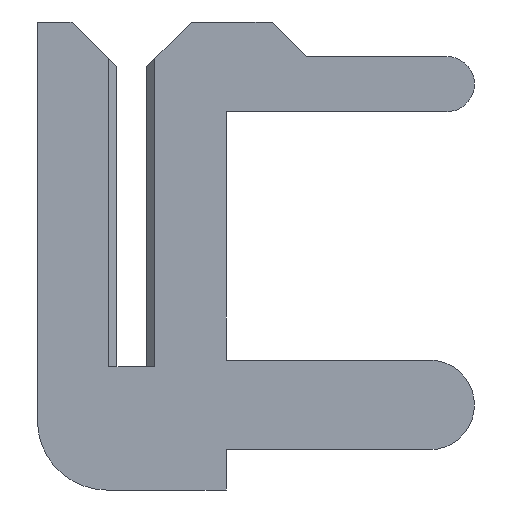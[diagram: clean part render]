
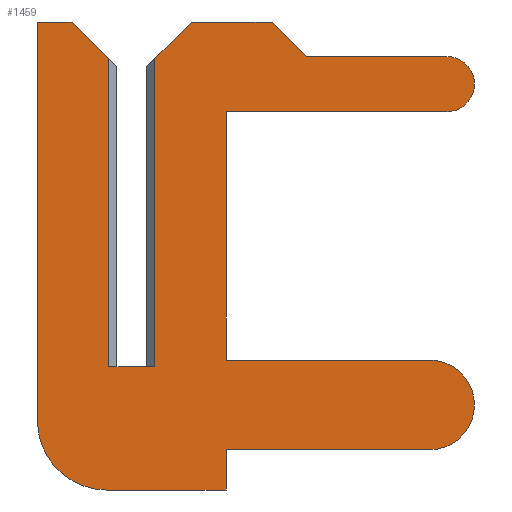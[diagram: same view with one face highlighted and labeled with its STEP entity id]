
A CAD part, left-side view. The second image highlights one B-rep face of the part: STEP entity #1459.
In plain terms, the highlighted planar face has unit normal (-1, 0, 0).
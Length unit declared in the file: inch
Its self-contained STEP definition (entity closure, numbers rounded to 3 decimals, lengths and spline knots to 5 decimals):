
#19 = ORIENTED_EDGE ( 'NONE', *, *, #220, .F. ) ;
#20 = CARTESIAN_POINT ( 'NONE',  ( -0.01, 0.01, 0. ) ) ;
#39 = CARTESIAN_POINT ( 'NONE',  ( -0.01, -0.1295, -0.0165 ) ) ;
#45 = VECTOR ( 'NONE', #202, 39.37008 ) ;
#55 = DIRECTION ( 'NONE',  ( 0., 0., 1. ) ) ;
#58 = ORIENTED_EDGE ( 'NONE', *, *, #839, .F. ) ;
#74 = EDGE_CURVE ( 'NONE', #909, #500, #1623, .T. ) ;
#92 = EDGE_CURVE ( 'NONE', #424, #322, #1539, .T. ) ;
#100 = VERTEX_POINT ( 'NONE', #1485 ) ;
#109 = CARTESIAN_POINT ( 'NONE',  ( -0.01, 0.0065, 0. ) ) ;
#128 = LINE ( 'NONE', #1517, #898 ) ;
#144 = VERTEX_POINT ( 'NONE', #276 ) ;
#150 = CARTESIAN_POINT ( 'NONE',  ( -0.01, 0.011, -0.0235 ) ) ;
#162 = VECTOR ( 'NONE', #884, 39.37008 ) ;
#175 = CARTESIAN_POINT ( 'NONE',  ( -0.01, -0.076, 0.135 ) ) ;
#179 = DIRECTION ( 'NONE',  ( 0., 0., -1. ) ) ;
#187 = EDGE_CURVE ( 'NONE', #1554, #996, #305, .T. ) ;
#195 = VECTOR ( 'NONE', #868, 39.37008 ) ;
#202 = DIRECTION ( 'NONE',  ( 0., -1., 0. ) ) ;
#220 = EDGE_CURVE ( 'NONE', #574, #391, #1400, .T. ) ;
#236 = VECTOR ( 'NONE', #342, 39.37008 ) ;
#249 = CARTESIAN_POINT ( 'NONE',  ( -0.01, 0.01, 0.134 ) ) ;
#250 = EDGE_CURVE ( 'NONE', #1470, #949, #1541, .T. ) ;
#256 = LINE ( 'NONE', #485, #236 ) ;
#273 = DIRECTION ( 'NONE',  ( 0., -0.707, -0.707 ) ) ;
#276 = CARTESIAN_POINT ( 'NONE',  ( -0.01, 0.026, 0.15 ) ) ;
#294 = DIRECTION ( 'NONE',  ( -1., 0., 0. ) ) ;
#298 = CARTESIAN_POINT ( 'NONE',  ( -0.01, -0.137, 0.123 ) ) ;
#305 = LINE ( 'NONE', #721, #1479 ) ;
#308 = DIRECTION ( 'NONE',  ( 0., 1., 0. ) ) ;
#322 = VERTEX_POINT ( 'NONE', #470 ) ;
#342 = DIRECTION ( 'NONE',  ( 0., -1., 0. ) ) ;
#343 = LINE ( 'NONE', #1061, #616 ) ;
#367 = LINE ( 'NONE', #109, #162 ) ;
#370 = EDGE_CURVE ( 'NONE', #996, #1699, #1678, .T. ) ;
#389 = ORIENTED_EDGE ( 'NONE', *, *, #857, .F. ) ;
#391 = VERTEX_POINT ( 'NONE', #599 ) ;
#394 = EDGE_CURVE ( 'NONE', #391, #1491, #128, .T. ) ;
#402 = VERTEX_POINT ( 'NONE', #175 ) ;
#406 = EDGE_CURVE ( 'NONE', #500, #1367, #1132, .T. ) ;
#419 = DIRECTION ( 'NONE',  ( 0., -0.707, -0.707 ) ) ;
#424 = VERTEX_POINT ( 'NONE', #1506 ) ;
#434 = LINE ( 'NONE', #876, #1455 ) ;
#441 = EDGE_CURVE ( 'NONE', #1434, #1015, #557, .T. ) ;
#447 = AXIS2_PLACEMENT_3D ( 'NONE', #1046, #1684, #1445 ) ;
#450 = DIRECTION ( 'NONE',  ( 0., 0., 1. ) ) ;
#451 = ORIENTED_EDGE ( 'NONE', *, *, #92, .T. ) ;
#470 = CARTESIAN_POINT ( 'NONE',  ( -0.01, -0.01, 0. ) ) ;
#485 = CARTESIAN_POINT ( 'NONE',  ( -0.01, -0.137, 0.135 ) ) ;
#500 = VERTEX_POINT ( 'NONE', #1148 ) ;
#511 = ORIENTED_EDGE ( 'NONE', *, *, #820, .F. ) ;
#533 = CARTESIAN_POINT ( 'NONE',  ( -0.01, -0.041, 0.003 ) ) ;
#551 = EDGE_CURVE ( 'NONE', #402, #909, #256, .T. ) ;
#557 = LINE ( 'NONE', #596, #195 ) ;
#558 = DIRECTION ( 'NONE',  ( 1., 0., 0. ) ) ;
#574 = VERTEX_POINT ( 'NONE', #1524 ) ;
#575 = CARTESIAN_POINT ( 'NONE',  ( -0.01, 0.011, -0.0535 ) ) ;
#595 = ORIENTED_EDGE ( 'NONE', *, *, #370, .F. ) ;
#596 = CARTESIAN_POINT ( 'NONE',  ( -0.01, -0.026, 0.15 ) ) ;
#599 = CARTESIAN_POINT ( 'NONE',  ( -0.01, -0.041, -0.0535 ) ) ;
#603 = AXIS2_PLACEMENT_3D ( 'NONE', #298, #558, #1094 ) ;
#610 = ORIENTED_EDGE ( 'NONE', *, *, #1169, .F. ) ;
#614 = VECTOR ( 'NONE', #1592, 39.37008 ) ;
#616 = VECTOR ( 'NONE', #273, 39.37008 ) ;
#641 = EDGE_LOOP ( 'NONE', ( #58, #451, #511, #794, #1536, #1165, #389, #1477, #869, #19, #690, #595, #672, #1370, #1292, #1181, #912, #610, #1146 ) ) ;
#655 = LINE ( 'NONE', #1009, #45 ) ;
#672 = ORIENTED_EDGE ( 'NONE', *, *, #187, .F. ) ;
#675 = CARTESIAN_POINT ( 'NONE',  ( -0.01, -0.041, -0.0535 ) ) ;
#677 = CARTESIAN_POINT ( 'NONE',  ( -0.01, -0.041, 0.003 ) ) ;
#690 = ORIENTED_EDGE ( 'NONE', *, *, #720, .F. ) ;
#698 = DIRECTION ( 'NONE',  ( 0., 1., 0. ) ) ;
#717 = LINE ( 'NONE', #1159, #855 ) ;
#720 = EDGE_CURVE ( 'NONE', #1699, #574, #434, .T. ) ;
#721 = CARTESIAN_POINT ( 'NONE',  ( -0.01, -0.1295, 0.003 ) ) ;
#759 = CARTESIAN_POINT ( 'NONE',  ( -0.01, -0.061, 0.15 ) ) ;
#765 = AXIS2_PLACEMENT_3D ( 'NONE', #39, #971, #450 ) ;
#773 = LINE ( 'NONE', #533, #1433 ) ;
#780 = EDGE_CURVE ( 'NONE', #100, #144, #655, .T. ) ;
#792 = LINE ( 'NONE', #922, #1275 ) ;
#794 = ORIENTED_EDGE ( 'NONE', *, *, #250, .T. ) ;
#801 = DIRECTION ( 'NONE',  ( 0., 0., -1. ) ) ;
#820 = EDGE_CURVE ( 'NONE', #1470, #322, #367, .T. ) ;
#839 = EDGE_CURVE ( 'NONE', #424, #1434, #717, .T. ) ;
#855 = VECTOR ( 'NONE', #1698, 39.37008 ) ;
#857 = EDGE_CURVE ( 'NONE', #1520, #100, #1025, .T. ) ;
#859 = DIRECTION ( 'NONE',  ( 0., 1., 0. ) ) ;
#868 = DIRECTION ( 'NONE',  ( 0., -1., 0. ) ) ;
#869 = ORIENTED_EDGE ( 'NONE', *, *, #394, .F. ) ;
#876 = CARTESIAN_POINT ( 'NONE',  ( -0.01, -0.041, -0.036 ) ) ;
#884 = DIRECTION ( 'NONE',  ( 0., -1., 0. ) ) ;
#898 = VECTOR ( 'NONE', #698, 39.37008 ) ;
#907 = DIRECTION ( 'NONE',  ( 0., 0., 1. ) ) ;
#909 = VERTEX_POINT ( 'NONE', #1551 ) ;
#912 = ORIENTED_EDGE ( 'NONE', *, *, #551, .F. ) ;
#922 = CARTESIAN_POINT ( 'NONE',  ( -0.01, -0.076, 0.135 ) ) ;
#935 = VECTOR ( 'NONE', #907, 39.37008 ) ;
#941 = CARTESIAN_POINT ( 'NONE',  ( -0.01, 0.041, -0.0235 ) ) ;
#947 = PLANE ( 'NONE',  #1156 ) ;
#949 = VERTEX_POINT ( 'NONE', #249 ) ;
#966 = VECTOR ( 'NONE', #308, 39.37008 ) ;
#971 = DIRECTION ( 'NONE',  ( 1., 0., 0. ) ) ;
#981 = CARTESIAN_POINT ( 'NONE',  ( -0.01, -0.041, 0.111 ) ) ;
#996 = VERTEX_POINT ( 'NONE', #1680 ) ;
#1008 = FACE_OUTER_BOUND ( 'NONE', #641, .T. ) ;
#1009 = CARTESIAN_POINT ( 'NONE',  ( -0.01, 0.026, 0.15 ) ) ;
#1015 = VERTEX_POINT ( 'NONE', #759 ) ;
#1025 = LINE ( 'NONE', #1557, #935 ) ;
#1046 = CARTESIAN_POINT ( 'NONE',  ( -0.01, 0.011, -0.0235 ) ) ;
#1047 = VECTOR ( 'NONE', #55, 39.37008 ) ;
#1050 = EDGE_CURVE ( 'NONE', #1491, #1520, #1208, .T. ) ;
#1061 = CARTESIAN_POINT ( 'NONE',  ( -0.01, 0.0065, 0.1305 ) ) ;
#1076 = CARTESIAN_POINT ( 'NONE',  ( -0.01, -0.01, 0.15 ) ) ;
#1090 = CARTESIAN_POINT ( 'NONE',  ( -0.01, -0.041, 0.111 ) ) ;
#1094 = DIRECTION ( 'NONE',  ( 0., 0., 1. ) ) ;
#1132 = LINE ( 'NONE', #981, #966 ) ;
#1142 = EDGE_CURVE ( 'NONE', #1367, #1554, #773, .T. ) ;
#1146 = ORIENTED_EDGE ( 'NONE', *, *, #441, .F. ) ;
#1148 = CARTESIAN_POINT ( 'NONE',  ( -0.01, -0.137, 0.111 ) ) ;
#1156 = AXIS2_PLACEMENT_3D ( 'NONE', #150, #294, #1482 ) ;
#1159 = CARTESIAN_POINT ( 'NONE',  ( -0.01, -0.0065, 0.1305 ) ) ;
#1165 = ORIENTED_EDGE ( 'NONE', *, *, #780, .F. ) ;
#1169 = EDGE_CURVE ( 'NONE', #1015, #402, #792, .T. ) ;
#1181 = ORIENTED_EDGE ( 'NONE', *, *, #74, .F. ) ;
#1208 = CIRCLE ( 'NONE', #447, 0.03 ) ;
#1224 = CARTESIAN_POINT ( 'NONE',  ( -0.01, -0.026, 0.15 ) ) ;
#1233 = CARTESIAN_POINT ( 'NONE',  ( -0.01, 0.01, -0.0235 ) ) ;
#1241 = DIRECTION ( 'NONE',  ( 0., -1., 0. ) ) ;
#1275 = VECTOR ( 'NONE', #419, 39.37008 ) ;
#1276 = VECTOR ( 'NONE', #179, 39.37008 ) ;
#1292 = ORIENTED_EDGE ( 'NONE', *, *, #406, .F. ) ;
#1367 = VERTEX_POINT ( 'NONE', #1090 ) ;
#1370 = ORIENTED_EDGE ( 'NONE', *, *, #1142, .F. ) ;
#1400 = LINE ( 'NONE', #675, #1276 ) ;
#1433 = VECTOR ( 'NONE', #801, 39.37008 ) ;
#1434 = VERTEX_POINT ( 'NONE', #1224 ) ;
#1445 = DIRECTION ( 'NONE',  ( 0., 0., 1. ) ) ;
#1455 = VECTOR ( 'NONE', #859, 39.37008 ) ;
#1459 = ADVANCED_FACE ( 'NONE', ( #1008 ), #947, .T. ) ;
#1470 = VERTEX_POINT ( 'NONE', #20 ) ;
#1477 = ORIENTED_EDGE ( 'NONE', *, *, #1050, .F. ) ;
#1479 = VECTOR ( 'NONE', #1241, 39.37008 ) ;
#1482 = DIRECTION ( 'NONE',  ( 0., 0., 1. ) ) ;
#1485 = CARTESIAN_POINT ( 'NONE',  ( -0.01, 0.041, 0.15 ) ) ;
#1491 = VERTEX_POINT ( 'NONE', #575 ) ;
#1503 = CARTESIAN_POINT ( 'NONE',  ( -0.01, -0.1295, -0.036 ) ) ;
#1506 = CARTESIAN_POINT ( 'NONE',  ( -0.01, -0.01, 0.134 ) ) ;
#1517 = CARTESIAN_POINT ( 'NONE',  ( -0.01, 0.011, -0.0535 ) ) ;
#1520 = VERTEX_POINT ( 'NONE', #941 ) ;
#1524 = CARTESIAN_POINT ( 'NONE',  ( -0.01, -0.041, -0.036 ) ) ;
#1536 = ORIENTED_EDGE ( 'NONE', *, *, #1625, .F. ) ;
#1539 = LINE ( 'NONE', #1076, #614 ) ;
#1541 = LINE ( 'NONE', #1233, #1047 ) ;
#1551 = CARTESIAN_POINT ( 'NONE',  ( -0.01, -0.137, 0.135 ) ) ;
#1554 = VERTEX_POINT ( 'NONE', #677 ) ;
#1557 = CARTESIAN_POINT ( 'NONE',  ( -0.01, 0.041, 0.15 ) ) ;
#1592 = DIRECTION ( 'NONE',  ( 0., 0., -1. ) ) ;
#1623 = CIRCLE ( 'NONE', #603, 0.012 ) ;
#1625 = EDGE_CURVE ( 'NONE', #144, #949, #343, .T. ) ;
#1678 = CIRCLE ( 'NONE', #765, 0.0195 ) ;
#1680 = CARTESIAN_POINT ( 'NONE',  ( -0.01, -0.1295, 0.003 ) ) ;
#1684 = DIRECTION ( 'NONE',  ( 1., 0., 0. ) ) ;
#1698 = DIRECTION ( 'NONE',  ( 0., -0.707, 0.707 ) ) ;
#1699 = VERTEX_POINT ( 'NONE', #1503 ) ;
